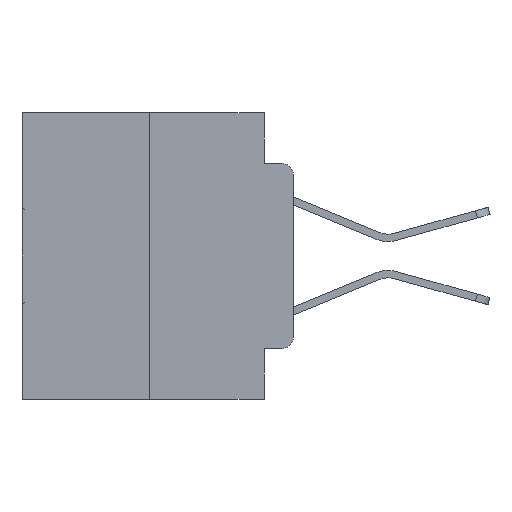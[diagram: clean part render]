
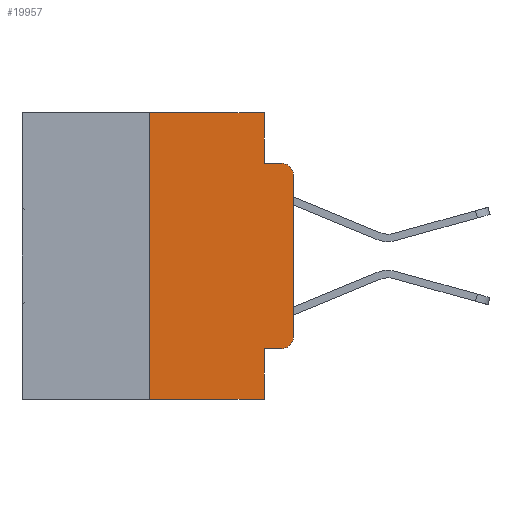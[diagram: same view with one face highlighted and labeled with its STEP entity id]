
A CAD part, left-side view. The second image highlights one B-rep face of the part: STEP entity #19957.
In plain terms, the highlighted planar face has unit normal (-1, 0, 0).
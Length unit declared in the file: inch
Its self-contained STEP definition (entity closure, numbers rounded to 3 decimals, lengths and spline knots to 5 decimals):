
#260 = CARTESIAN_POINT ( 'NONE',  ( 0., 0.051, -0.4115 ) ) ;
#510 = VECTOR ( 'NONE', #4916, 39.37008 ) ;
#1086 = VERTEX_POINT ( 'NONE', #2164 ) ;
#1828 = DIRECTION ( 'NONE',  ( 0., -1., 0. ) ) ;
#2039 = CARTESIAN_POINT ( 'NONE',  ( 0., 0.473, 0. ) ) ;
#2164 = CARTESIAN_POINT ( 'NONE',  ( 0., 0.051, -0.5 ) ) ;
#2636 = CARTESIAN_POINT ( 'NONE',  ( 0., 0., 0. ) ) ;
#2649 = CARTESIAN_POINT ( 'NONE',  ( 0., 0.051, 0. ) ) ;
#3232 = CARTESIAN_POINT ( 'NONE',  ( 0., 0.25, 0. ) ) ;
#4672 = DIRECTION ( 'NONE',  ( 0., 0., -1. ) ) ;
#4704 = CARTESIAN_POINT ( 'NONE',  ( 0., 0.473, -0.5 ) ) ;
#4916 = DIRECTION ( 'NONE',  ( 0., 0., -1. ) ) ;
#5420 = AXIS2_PLACEMENT_3D ( 'NONE', #5708, #10066, #19841 ) ;
#5708 = CARTESIAN_POINT ( 'NONE',  ( 0., 0.02, -0.3915 ) ) ;
#5960 = ORIENTED_EDGE ( 'NONE', *, *, #9539, .T. ) ;
#6229 = VERTEX_POINT ( 'NONE', #27786 ) ;
#6256 = CARTESIAN_POINT ( 'NONE',  ( 0., 0.473, 0. ) ) ;
#6483 = DIRECTION ( 'NONE',  ( 0., -1., 0. ) ) ;
#6999 = LINE ( 'NONE', #19528, #510 ) ;
#7963 = VERTEX_POINT ( 'NONE', #260 ) ;
#8108 = LINE ( 'NONE', #4704, #19718 ) ;
#8484 = DIRECTION ( 'NONE',  ( 0., 0., 1. ) ) ;
#9539 = EDGE_CURVE ( 'NONE', #7963, #29672, #15817, .T. ) ;
#9554 = CARTESIAN_POINT ( 'NONE',  ( 0., 0., -0.3915 ) ) ;
#10066 = DIRECTION ( 'NONE',  ( -1., 0., 0. ) ) ;
#10518 = ORIENTED_EDGE ( 'NONE', *, *, #29758, .F. ) ;
#10821 = VERTEX_POINT ( 'NONE', #28074 ) ;
#11219 = EDGE_LOOP ( 'NONE', ( #18097, #30696, #22433, #10518, #26188, #28333, #30122, #27005, #5960, #22206 ) ) ;
#12197 = DIRECTION ( 'NONE',  ( 0., 0., -1. ) ) ;
#12242 = EDGE_CURVE ( 'NONE', #10821, #23182, #25715, .T. ) ;
#13558 = VERTEX_POINT ( 'NONE', #29992 ) ;
#14521 = VECTOR ( 'NONE', #8484, 39.37008 ) ;
#14908 = AXIS2_PLACEMENT_3D ( 'NONE', #26845, #27476, #12197 ) ;
#15149 = CIRCLE ( 'NONE', #5420, 0.02 ) ;
#15169 = DIRECTION ( 'NONE',  ( 0., 0., 1. ) ) ;
#15675 = DIRECTION ( 'NONE',  ( 0., -1., 0. ) ) ;
#15817 = LINE ( 'NONE', #28688, #19499 ) ;
#16021 = DIRECTION ( 'NONE',  ( 1., 0., 0. ) ) ;
#16473 = DIRECTION ( 'NONE',  ( 0., -1., 0. ) ) ;
#17587 = VECTOR ( 'NONE', #15675, 39.37008 ) ;
#18097 = ORIENTED_EDGE ( 'NONE', *, *, #26500, .T. ) ;
#18383 = VERTEX_POINT ( 'NONE', #24588 ) ;
#18431 = FACE_OUTER_BOUND ( 'NONE', #11219, .T. ) ;
#18762 = EDGE_CURVE ( 'NONE', #23182, #29693, #18895, .T. ) ;
#18895 = LINE ( 'NONE', #2039, #28621 ) ;
#19499 = VECTOR ( 'NONE', #1828, 39.37008 ) ;
#19528 = CARTESIAN_POINT ( 'NONE',  ( 0., 0.051, 0. ) ) ;
#19718 = VECTOR ( 'NONE', #6483, 39.37008 ) ;
#19841 = DIRECTION ( 'NONE',  ( 0., 0., -1. ) ) ;
#19957 = ADVANCED_FACE ( 'NONE', ( #18431 ), #28280, .F. ) ;
#20337 = EDGE_CURVE ( 'NONE', #6229, #13558, #30974, .T. ) ;
#20824 = CARTESIAN_POINT ( 'NONE',  ( 0., 0.051, -0.0885 ) ) ;
#21387 = AXIS2_PLACEMENT_3D ( 'NONE', #6256, #16021, #26670 ) ;
#22206 = ORIENTED_EDGE ( 'NONE', *, *, #24052, .T. ) ;
#22433 = ORIENTED_EDGE ( 'NONE', *, *, #20337, .F. ) ;
#22903 = EDGE_CURVE ( 'NONE', #10821, #1086, #8108, .T. ) ;
#23182 = VERTEX_POINT ( 'NONE', #3232 ) ;
#23269 = VECTOR ( 'NONE', #15169, 39.37008 ) ;
#23596 = EDGE_CURVE ( 'NONE', #7963, #1086, #25354, .T. ) ;
#24052 = EDGE_CURVE ( 'NONE', #29672, #29330, #15149, .T. ) ;
#24588 = CARTESIAN_POINT ( 'NONE',  ( 0., 0., -0.1085 ) ) ;
#24763 = CARTESIAN_POINT ( 'NONE',  ( 0., 0.051, 0. ) ) ;
#25354 = LINE ( 'NONE', #24763, #25922 ) ;
#25715 = LINE ( 'NONE', #30704, #14521 ) ;
#25922 = VECTOR ( 'NONE', #4672, 39.37008 ) ;
#26188 = ORIENTED_EDGE ( 'NONE', *, *, #18762, .F. ) ;
#26222 = CIRCLE ( 'NONE', #14908, 0.02 ) ;
#26500 = EDGE_CURVE ( 'NONE', #29330, #18383, #31764, .T. ) ;
#26670 = DIRECTION ( 'NONE',  ( 0., 0., -1. ) ) ;
#26845 = CARTESIAN_POINT ( 'NONE',  ( 0., 0.02, -0.1085 ) ) ;
#27005 = ORIENTED_EDGE ( 'NONE', *, *, #23596, .F. ) ;
#27476 = DIRECTION ( 'NONE',  ( -1., 0., 0. ) ) ;
#27786 = CARTESIAN_POINT ( 'NONE',  ( 0., 0.051, -0.0885 ) ) ;
#28074 = CARTESIAN_POINT ( 'NONE',  ( 0., 0.25, -0.5 ) ) ;
#28280 = PLANE ( 'NONE',  #21387 ) ;
#28333 = ORIENTED_EDGE ( 'NONE', *, *, #12242, .F. ) ;
#28621 = VECTOR ( 'NONE', #16473, 39.37008 ) ;
#28688 = CARTESIAN_POINT ( 'NONE',  ( 0., 0.051, -0.4115 ) ) ;
#29203 = CARTESIAN_POINT ( 'NONE',  ( 0., 0.02, -0.4115 ) ) ;
#29330 = VERTEX_POINT ( 'NONE', #9554 ) ;
#29672 = VERTEX_POINT ( 'NONE', #29203 ) ;
#29693 = VERTEX_POINT ( 'NONE', #2649 ) ;
#29758 = EDGE_CURVE ( 'NONE', #29693, #6229, #6999, .T. ) ;
#29992 = CARTESIAN_POINT ( 'NONE',  ( 0., 0.02, -0.0885 ) ) ;
#30122 = ORIENTED_EDGE ( 'NONE', *, *, #22903, .T. ) ;
#30589 = EDGE_CURVE ( 'NONE', #18383, #13558, #26222, .T. ) ;
#30696 = ORIENTED_EDGE ( 'NONE', *, *, #30589, .T. ) ;
#30704 = CARTESIAN_POINT ( 'NONE',  ( 0., 0.25, 0. ) ) ;
#30974 = LINE ( 'NONE', #20824, #17587 ) ;
#31764 = LINE ( 'NONE', #2636, #23269 ) ;
